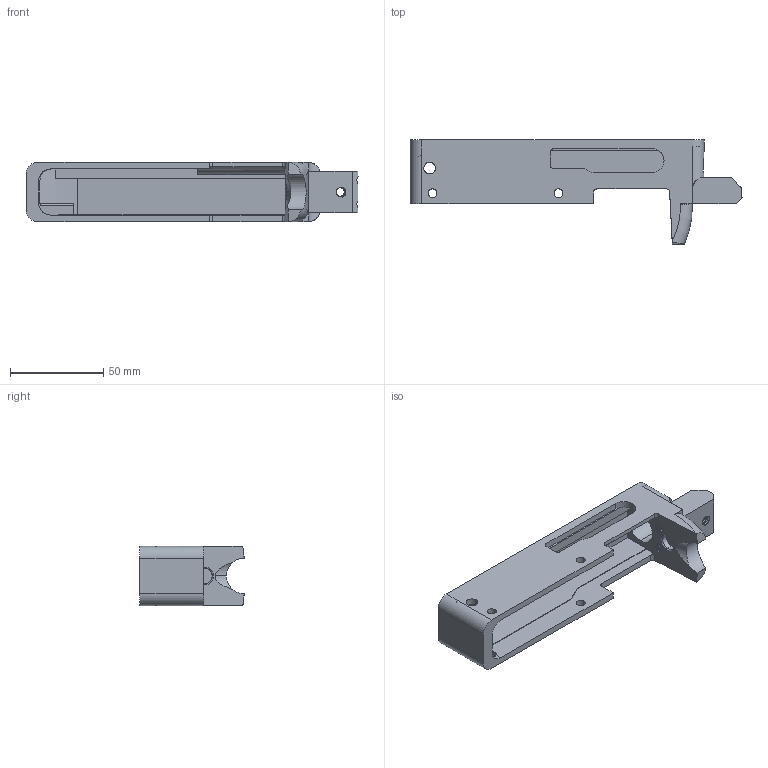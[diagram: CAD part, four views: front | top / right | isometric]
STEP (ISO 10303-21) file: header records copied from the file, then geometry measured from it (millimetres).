
FILE_DESCRIPTION (( 'STEP AP214' ), '1' );
FILE_NAME ('10-22 Receiver Flat Top B1.STEP', '2015-05-12T21:31:50', ( 'WarFairy' ), ( '' ), 'SwSTEP 2.0', 'SolidWorks 2015', '' );
FILE_SCHEMA (( 'AUTOMOTIVE_DESIGN' ));
Length unit declared in the file: inch
Products named in the file (1): 10-22 Receiver Flat Top B1
Bounding box: 177.8 x 55.93 x 31.75 mm (x, y, z)
Volume: 70544.1 mm3; surface area: 35551 mm2
Topology: 1 solids, 1 shells, 242 faces, 723 edges, 478 vertices
Faces by surface type: cylinder 158, plane 65, bspline 12, torus 7
Entity records: 15807 total; most frequent: CARTESIAN_POINT 9972, ORIENTED_EDGE 1442, DIRECTION 985, EDGE_CURVE 721, VERTEX_POINT 478, AXIS2_PLACEMENT_3D 335, VECTOR 315, LINE 315
